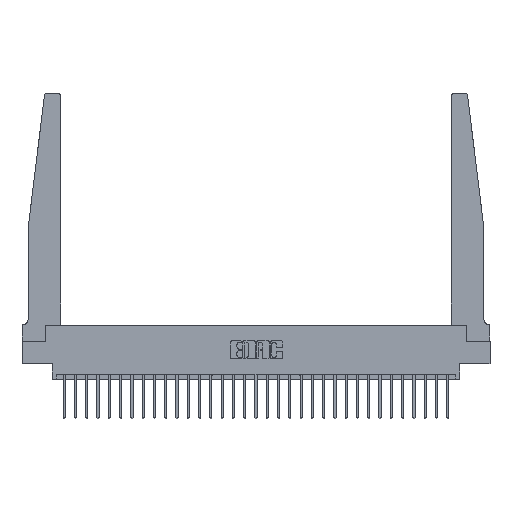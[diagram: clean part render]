
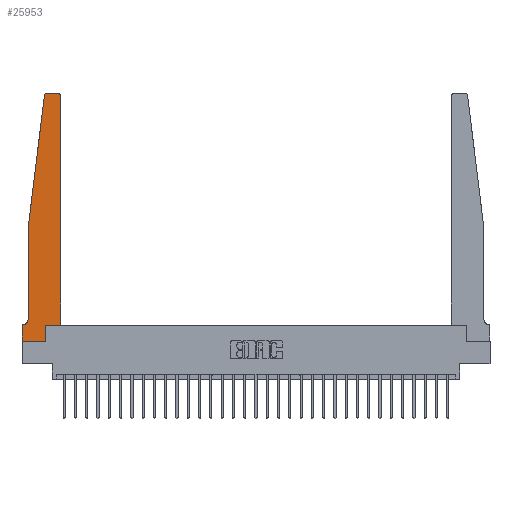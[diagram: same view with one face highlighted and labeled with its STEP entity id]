
A CAD part, top view. The second image highlights one B-rep face of the part: STEP entity #25953.
In plain terms, the highlighted planar face has unit normal (0, 0, 1).
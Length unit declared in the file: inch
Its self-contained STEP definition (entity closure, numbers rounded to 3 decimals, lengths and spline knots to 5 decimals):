
#386 = VECTOR ( 'NONE', #27325, 39.37008 ) ;
#1589 = CARTESIAN_POINT ( 'NONE',  ( 0.2605, 0.18, 0.37 ) ) ;
#1781 = ORIENTED_EDGE ( 'NONE', *, *, #12649, .T. ) ;
#1788 = CARTESIAN_POINT ( 'NONE',  ( 0.24675, 2.72367, 0.37 ) ) ;
#1922 = AXIS2_PLACEMENT_3D ( 'NONE', #22157, #8749, #1970 ) ;
#1970 = DIRECTION ( 'NONE',  ( 1., 0., 0. ) ) ;
#2793 = DIRECTION ( 'NONE',  ( -1., 0., 0. ) ) ;
#2847 = VERTEX_POINT ( 'NONE', #12249 ) ;
#3905 = VECTOR ( 'NONE', #5943, 39.37008 ) ;
#4012 = EDGE_CURVE ( 'NONE', #27741, #14967, #17742, .T. ) ;
#4169 = PLANE ( 'NONE',  #1922 ) ;
#4176 = DIRECTION ( 'NONE',  ( 0., 0., 1. ) ) ;
#4443 = EDGE_CURVE ( 'NONE', #5134, #16072, #27579, .T. ) ;
#4613 = CARTESIAN_POINT ( 'NONE',  ( 0.065, 1.25, 0.37 ) ) ;
#4701 = DIRECTION ( 'NONE',  ( 1., 0., 0. ) ) ;
#5134 = VERTEX_POINT ( 'NONE', #26748 ) ;
#5562 = LINE ( 'NONE', #26223, #10355 ) ;
#5622 = LINE ( 'NONE', #25711, #19350 ) ;
#5943 = DIRECTION ( 'NONE',  ( 0., 1., 0. ) ) ;
#6181 = CIRCLE ( 'NONE', #23601, 0.03 ) ;
#7533 = AXIS2_PLACEMENT_3D ( 'NONE', #21100, #12232, #12093 ) ;
#8067 = DIRECTION ( 'NONE',  ( -1., 0., 0. ) ) ;
#8363 = VECTOR ( 'NONE', #10588, 39.37008 ) ;
#8466 = ORIENTED_EDGE ( 'NONE', *, *, #16114, .T. ) ;
#8622 = CARTESIAN_POINT ( 'NONE',  ( 0.425, 2.72, 0.37 ) ) ;
#8674 = CARTESIAN_POINT ( 'NONE',  ( 0.2605, 0., 0.37 ) ) ;
#8749 = DIRECTION ( 'NONE',  ( 0., 0., 1. ) ) ;
#9353 = EDGE_CURVE ( 'NONE', #16072, #27741, #20301, .T. ) ;
#9451 = CARTESIAN_POINT ( 'NONE',  ( 0.015, 0.1875, 0.37 ) ) ;
#9869 = VERTEX_POINT ( 'NONE', #9451 ) ;
#9957 = CARTESIAN_POINT ( 'NONE',  ( 0.425, 0.18, 0.37 ) ) ;
#10355 = VECTOR ( 'NONE', #8067, 39.37008 ) ;
#10588 = DIRECTION ( 'NONE',  ( 0., -1., 0. ) ) ;
#10705 = VECTOR ( 'NONE', #25060, 39.37008 ) ;
#10951 = CARTESIAN_POINT ( 'NONE',  ( 0., 0., 0.37 ) ) ;
#12093 = DIRECTION ( 'NONE',  ( -1., 0., 0. ) ) ;
#12119 = ORIENTED_EDGE ( 'NONE', *, *, #27842, .T. ) ;
#12232 = DIRECTION ( 'NONE',  ( 0., 0., -1. ) ) ;
#12249 = CARTESIAN_POINT ( 'NONE',  ( 0.065, 0.2375, 0.37 ) ) ;
#12360 = EDGE_LOOP ( 'NONE', ( #27511, #21555, #13219, #8466, #14533, #25301, #28707, #1781, #25568, #25315, #19495, #12119 ) ) ;
#12649 = EDGE_CURVE ( 'NONE', #24988, #14506, #21852, .T. ) ;
#12941 = CARTESIAN_POINT ( 'NONE',  ( 0.065, 1.25, 0.37 ) ) ;
#13219 = ORIENTED_EDGE ( 'NONE', *, *, #4012, .T. ) ;
#13364 = VERTEX_POINT ( 'NONE', #1589 ) ;
#14506 = VERTEX_POINT ( 'NONE', #8674 ) ;
#14533 = ORIENTED_EDGE ( 'NONE', *, *, #24729, .T. ) ;
#14967 = VERTEX_POINT ( 'NONE', #4613 ) ;
#15009 = LINE ( 'NONE', #15238, #8363 ) ;
#15238 = CARTESIAN_POINT ( 'NONE',  ( 0., 0., 0.37 ) ) ;
#15479 = VECTOR ( 'NONE', #2793, 39.37008 ) ;
#15898 = CARTESIAN_POINT ( 'NONE',  ( 0., 0., 0.37 ) ) ;
#16072 = VERTEX_POINT ( 'NONE', #17243 ) ;
#16114 = EDGE_CURVE ( 'NONE', #14967, #2847, #26244, .T. ) ;
#17030 = LINE ( 'NONE', #17170, #3905 ) ;
#17170 = CARTESIAN_POINT ( 'NONE',  ( 0.425, 0.18, 0.37 ) ) ;
#17243 = CARTESIAN_POINT ( 'NONE',  ( 0.27653, 2.75, 0.37 ) ) ;
#17460 = AXIS2_PLACEMENT_3D ( 'NONE', #17908, #4176, #22163 ) ;
#17742 = LINE ( 'NONE', #22277, #386 ) ;
#17908 = CARTESIAN_POINT ( 'NONE',  ( 0.27653, 2.72, 0.37 ) ) ;
#17978 = VERTEX_POINT ( 'NONE', #8622 ) ;
#18161 = VERTEX_POINT ( 'NONE', #9957 ) ;
#18718 = LINE ( 'NONE', #27869, #10705 ) ;
#18768 = DIRECTION ( 'NONE',  ( 0., 1., 0. ) ) ;
#18823 = EDGE_CURVE ( 'NONE', #21595, #24988, #15009, .T. ) ;
#19111 = VECTOR ( 'NONE', #19667, 39.37008 ) ;
#19163 = DIRECTION ( 'NONE',  ( 0., -1., 0. ) ) ;
#19350 = VECTOR ( 'NONE', #18768, 39.37008 ) ;
#19495 = ORIENTED_EDGE ( 'NONE', *, *, #22331, .T. ) ;
#19667 = DIRECTION ( 'NONE',  ( 1., 0., 0. ) ) ;
#19870 = EDGE_CURVE ( 'NONE', #13364, #18161, #18718, .T. ) ;
#20124 = FACE_OUTER_BOUND ( 'NONE', #12360, .T. ) ;
#20301 = CIRCLE ( 'NONE', #17460, 0.03 ) ;
#20717 = CIRCLE ( 'NONE', #7533, 0.05 ) ;
#21100 = CARTESIAN_POINT ( 'NONE',  ( 0.015, 0.2375, 0.37 ) ) ;
#21555 = ORIENTED_EDGE ( 'NONE', *, *, #9353, .T. ) ;
#21595 = VERTEX_POINT ( 'NONE', #28772 ) ;
#21852 = LINE ( 'NONE', #10951, #19111 ) ;
#22157 = CARTESIAN_POINT ( 'NONE',  ( 0., 0.1875, 0.37 ) ) ;
#22163 = DIRECTION ( 'NONE',  ( 1., 0., 0. ) ) ;
#22277 = CARTESIAN_POINT ( 'NONE',  ( 0.065, 1.25, 0.37 ) ) ;
#22331 = EDGE_CURVE ( 'NONE', #18161, #17978, #17030, .T. ) ;
#22412 = DIRECTION ( 'NONE',  ( 0., 0., 1. ) ) ;
#22549 = CARTESIAN_POINT ( 'NONE',  ( 0.395, 2.72, 0.37 ) ) ;
#23601 = AXIS2_PLACEMENT_3D ( 'NONE', #22549, #22412, #4701 ) ;
#24016 = EDGE_CURVE ( 'NONE', #9869, #21595, #5562, .T. ) ;
#24729 = EDGE_CURVE ( 'NONE', #2847, #9869, #20717, .T. ) ;
#24988 = VERTEX_POINT ( 'NONE', #15898 ) ;
#25060 = DIRECTION ( 'NONE',  ( 1., 0., 0. ) ) ;
#25301 = ORIENTED_EDGE ( 'NONE', *, *, #24016, .T. ) ;
#25315 = ORIENTED_EDGE ( 'NONE', *, *, #19870, .T. ) ;
#25568 = ORIENTED_EDGE ( 'NONE', *, *, #27583, .T. ) ;
#25711 = CARTESIAN_POINT ( 'NONE',  ( 0.2605, 0.18, 0.37 ) ) ;
#25810 = VECTOR ( 'NONE', #19163, 39.37008 ) ;
#25953 = ADVANCED_FACE ( 'NONE', ( #20124 ), #4169, .T. ) ;
#26223 = CARTESIAN_POINT ( 'NONE',  ( 0.065, 0.1875, 0.37 ) ) ;
#26244 = LINE ( 'NONE', #12941, #25810 ) ;
#26748 = CARTESIAN_POINT ( 'NONE',  ( 0.395, 2.75, 0.37 ) ) ;
#27149 = CARTESIAN_POINT ( 'NONE',  ( 0.25, 2.75, 0.37 ) ) ;
#27325 = DIRECTION ( 'NONE',  ( -0.122, -0.992, 0. ) ) ;
#27511 = ORIENTED_EDGE ( 'NONE', *, *, #4443, .T. ) ;
#27579 = LINE ( 'NONE', #27149, #15479 ) ;
#27583 = EDGE_CURVE ( 'NONE', #14506, #13364, #5622, .T. ) ;
#27741 = VERTEX_POINT ( 'NONE', #1788 ) ;
#27842 = EDGE_CURVE ( 'NONE', #17978, #5134, #6181, .T. ) ;
#27869 = CARTESIAN_POINT ( 'NONE',  ( 0.425, 0.18, 0.37 ) ) ;
#28707 = ORIENTED_EDGE ( 'NONE', *, *, #18823, .T. ) ;
#28772 = CARTESIAN_POINT ( 'NONE',  ( 0., 0.1875, 0.37 ) ) ;
